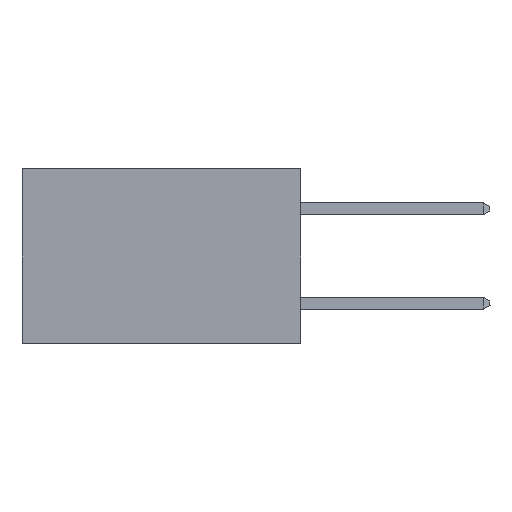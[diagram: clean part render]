
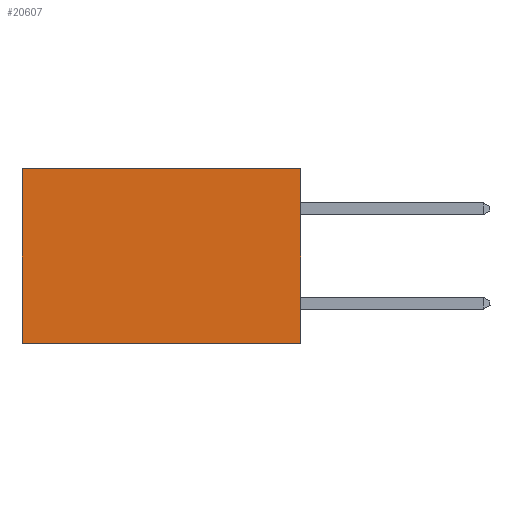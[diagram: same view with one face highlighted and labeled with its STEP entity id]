
A CAD part, left-side view. The second image highlights one B-rep face of the part: STEP entity #20607.
In plain terms, the highlighted planar face has unit normal (-1, 0, 0).
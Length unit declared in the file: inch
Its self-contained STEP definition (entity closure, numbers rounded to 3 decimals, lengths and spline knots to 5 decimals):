
#265 = EDGE_LOOP ( 'NONE', ( #6484, #28310, #26005, #480 ) ) ;
#383 = VECTOR ( 'NONE', #22943, 39.37008 ) ;
#480 = ORIENTED_EDGE ( 'NONE', *, *, #16402, .T. ) ;
#596 = CARTESIAN_POINT ( 'NONE',  ( 0.277, 0., 0. ) ) ;
#962 = VECTOR ( 'NONE', #17529, 39.37008 ) ;
#1806 = LINE ( 'NONE', #2271, #962 ) ;
#2271 = CARTESIAN_POINT ( 'NONE',  ( 0.277, 0., -0.37 ) ) ;
#4249 = VERTEX_POINT ( 'NONE', #4462 ) ;
#4462 = CARTESIAN_POINT ( 'NONE',  ( 0.277, 0.59, -0.37 ) ) ;
#5185 = VECTOR ( 'NONE', #21819, 39.37008 ) ;
#5636 = EDGE_CURVE ( 'NONE', #20860, #4249, #26229, .T. ) ;
#6484 = ORIENTED_EDGE ( 'NONE', *, *, #19610, .T. ) ;
#7023 = FACE_OUTER_BOUND ( 'NONE', #265, .T. ) ;
#7722 = CARTESIAN_POINT ( 'NONE',  ( 0.277, 0., 0. ) ) ;
#10177 = CARTESIAN_POINT ( 'NONE',  ( 0.277, 0.59, 0. ) ) ;
#11971 = VERTEX_POINT ( 'NONE', #10177 ) ;
#15052 = EDGE_CURVE ( 'NONE', #30623, #20860, #1806, .T. ) ;
#15081 = AXIS2_PLACEMENT_3D ( 'NONE', #29934, #32411, #17475 ) ;
#16402 = EDGE_CURVE ( 'NONE', #30623, #11971, #20083, .T. ) ;
#16679 = VECTOR ( 'NONE', #31396, 39.37008 ) ;
#17475 = DIRECTION ( 'NONE',  ( 0., 0., -1. ) ) ;
#17529 = DIRECTION ( 'NONE',  ( 0., 0., -1. ) ) ;
#18263 = LINE ( 'NONE', #26425, #16679 ) ;
#19610 = EDGE_CURVE ( 'NONE', #11971, #4249, #18263, .T. ) ;
#20083 = LINE ( 'NONE', #7722, #383 ) ;
#20607 = ADVANCED_FACE ( 'NONE', ( #7023 ), #22429, .F. ) ;
#20860 = VERTEX_POINT ( 'NONE', #30902 ) ;
#21819 = DIRECTION ( 'NONE',  ( 0., 1., 0. ) ) ;
#21934 = CARTESIAN_POINT ( 'NONE',  ( 0.277, 0., -0.37 ) ) ;
#22429 = PLANE ( 'NONE',  #15081 ) ;
#22943 = DIRECTION ( 'NONE',  ( 0., 1., 0. ) ) ;
#26005 = ORIENTED_EDGE ( 'NONE', *, *, #15052, .F. ) ;
#26229 = LINE ( 'NONE', #21934, #5185 ) ;
#26425 = CARTESIAN_POINT ( 'NONE',  ( 0.277, 0.59, -0.37 ) ) ;
#28310 = ORIENTED_EDGE ( 'NONE', *, *, #5636, .F. ) ;
#29934 = CARTESIAN_POINT ( 'NONE',  ( 0.277, 0., -0.37 ) ) ;
#30623 = VERTEX_POINT ( 'NONE', #596 ) ;
#30902 = CARTESIAN_POINT ( 'NONE',  ( 0.277, 0., -0.37 ) ) ;
#31396 = DIRECTION ( 'NONE',  ( 0., 0., -1. ) ) ;
#32411 = DIRECTION ( 'NONE',  ( 1., 0., 0. ) ) ;
